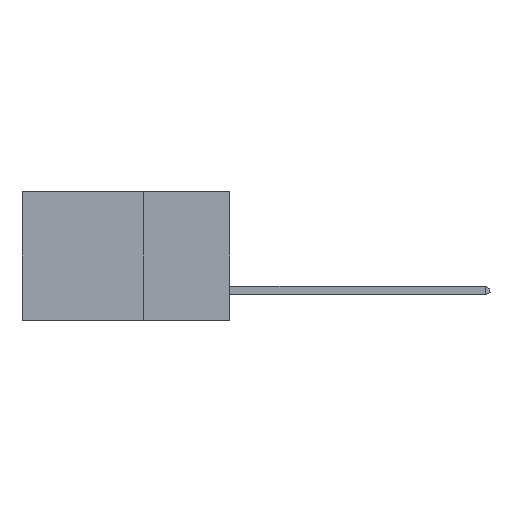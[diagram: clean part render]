
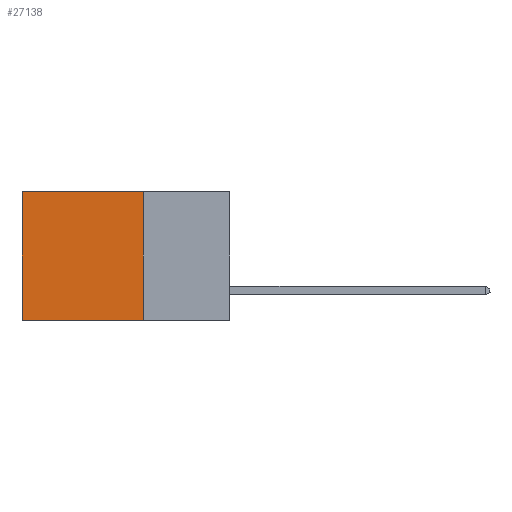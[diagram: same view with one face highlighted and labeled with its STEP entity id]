
A CAD part, left-side view. The second image highlights one B-rep face of the part: STEP entity #27138.
In plain terms, the highlighted planar face has unit normal (-1, 0, 0).
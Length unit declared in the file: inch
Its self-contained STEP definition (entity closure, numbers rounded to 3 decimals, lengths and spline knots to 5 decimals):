
#3862 = ORIENTED_EDGE ( 'NONE', *, *, #17472, .T. ) ;
#3985 = EDGE_CURVE ( 'NONE', #4386, #26216, #13765, .T. ) ;
#4386 = VERTEX_POINT ( 'NONE', #11121 ) ;
#5871 = DIRECTION ( 'NONE',  ( 0., 0., -1. ) ) ;
#6262 = LINE ( 'NONE', #19310, #27374 ) ;
#6452 = CARTESIAN_POINT ( 'NONE',  ( 0.298, 0.6, -0.37 ) ) ;
#6510 = CARTESIAN_POINT ( 'NONE',  ( 0.298, 0.6, 0. ) ) ;
#7480 = VERTEX_POINT ( 'NONE', #6452 ) ;
#7772 = VECTOR ( 'NONE', #14940, 39.37008 ) ;
#7930 = VERTEX_POINT ( 'NONE', #8006 ) ;
#8006 = CARTESIAN_POINT ( 'NONE',  ( 0.298, 0.25, -0.37 ) ) ;
#10205 = CARTESIAN_POINT ( 'NONE',  ( 0.298, 0.6, 0. ) ) ;
#10749 = VECTOR ( 'NONE', #16212, 39.37008 ) ;
#11121 = CARTESIAN_POINT ( 'NONE',  ( 0.298, 0.25, 0. ) ) ;
#11905 = EDGE_LOOP ( 'NONE', ( #3862, #17044, #23450, #17345 ) ) ;
#13765 = LINE ( 'NONE', #25489, #7772 ) ;
#14421 = CARTESIAN_POINT ( 'NONE',  ( 0.298, 0.25, 0. ) ) ;
#14657 = EDGE_CURVE ( 'NONE', #4386, #7930, #23053, .T. ) ;
#14720 = AXIS2_PLACEMENT_3D ( 'NONE', #14421, #21010, #16882 ) ;
#14940 = DIRECTION ( 'NONE',  ( 0., 1., 0. ) ) ;
#16025 = CARTESIAN_POINT ( 'NONE',  ( 0.298, 0.25, 0. ) ) ;
#16212 = DIRECTION ( 'NONE',  ( 0., 0., -1. ) ) ;
#16882 = DIRECTION ( 'NONE',  ( 0., 0., -1. ) ) ;
#17044 = ORIENTED_EDGE ( 'NONE', *, *, #23976, .F. ) ;
#17345 = ORIENTED_EDGE ( 'NONE', *, *, #3985, .T. ) ;
#17472 = EDGE_CURVE ( 'NONE', #26216, #7480, #25567, .T. ) ;
#19020 = PLANE ( 'NONE',  #14720 ) ;
#19310 = CARTESIAN_POINT ( 'NONE',  ( 0.298, 0.25, -0.37 ) ) ;
#21010 = DIRECTION ( 'NONE',  ( 1., 0., 0. ) ) ;
#21577 = DIRECTION ( 'NONE',  ( 0., 1., 0. ) ) ;
#23053 = LINE ( 'NONE', #16025, #10749 ) ;
#23450 = ORIENTED_EDGE ( 'NONE', *, *, #14657, .F. ) ;
#23976 = EDGE_CURVE ( 'NONE', #7930, #7480, #6262, .T. ) ;
#25489 = CARTESIAN_POINT ( 'NONE',  ( 0.298, 0.25, 0. ) ) ;
#25567 = LINE ( 'NONE', #10205, #26993 ) ;
#26216 = VERTEX_POINT ( 'NONE', #6510 ) ;
#26993 = VECTOR ( 'NONE', #5871, 39.37008 ) ;
#27138 = ADVANCED_FACE ( 'NONE', ( #27770 ), #19020, .F. ) ;
#27374 = VECTOR ( 'NONE', #21577, 39.37008 ) ;
#27770 = FACE_OUTER_BOUND ( 'NONE', #11905, .T. ) ;
